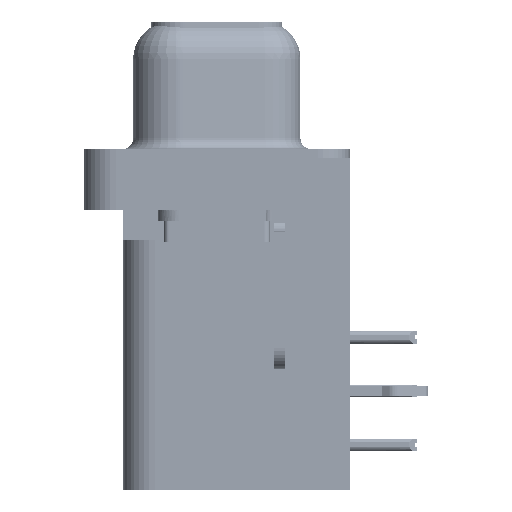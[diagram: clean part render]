
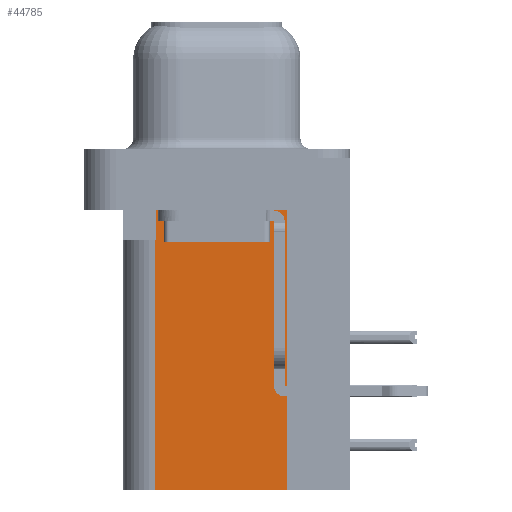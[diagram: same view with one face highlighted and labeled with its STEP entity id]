
A CAD part, left-side view. The second image highlights one B-rep face of the part: STEP entity #44785.
In plain terms, the highlighted planar face has unit normal (-1, 0, 0).
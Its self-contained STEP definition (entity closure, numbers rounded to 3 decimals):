
#141 = AXIS2_PLACEMENT_3D ( 'NONE', #15658, #43529, #22673 ) ;
#3928 = DIRECTION ( 'NONE',  ( 0., 0., -1. ) ) ;
#4712 = DIRECTION ( 'NONE',  ( 0., 1., 0. ) ) ;
#4950 = VERTEX_POINT ( 'NONE', #34825 ) ;
#5890 = VECTOR ( 'NONE', #4712, 1000. ) ;
#6007 = VERTEX_POINT ( 'NONE', #10439 ) ;
#7866 = VERTEX_POINT ( 'NONE', #42041 ) ;
#8659 = LINE ( 'NONE', #20892, #18112 ) ;
#9629 = VERTEX_POINT ( 'NONE', #35778 ) ;
#10373 = ORIENTED_EDGE ( 'NONE', *, *, #26933, .T. ) ;
#10439 = CARTESIAN_POINT ( 'NONE',  ( 3.7, 2.895, -2.5 ) ) ;
#11635 = ORIENTED_EDGE ( 'NONE', *, *, #17318, .F. ) ;
#14782 = DIRECTION ( 'NONE',  ( 0., 1., 0. ) ) ;
#15658 = CARTESIAN_POINT ( 'NONE',  ( 3.7, -3.295, -15.7 ) ) ;
#16443 = LINE ( 'NONE', #43155, #5890 ) ;
#17318 = EDGE_CURVE ( 'NONE', #39804, #7866, #29363, .T. ) ;
#18112 = VECTOR ( 'NONE', #24385, 1000. ) ;
#18471 = ORIENTED_EDGE ( 'NONE', *, *, #22026, .T. ) ;
#19709 = VERTEX_POINT ( 'NONE', #25053 ) ;
#20469 = EDGE_LOOP ( 'NONE', ( #25686, #10373, #35049, #11635, #25827, #18471 ) ) ;
#20892 = CARTESIAN_POINT ( 'NONE',  ( 3.7, -3.295, -2.5 ) ) ;
#21402 = CARTESIAN_POINT ( 'NONE',  ( 3.7, 2.925, -15.7 ) ) ;
#21564 = EDGE_CURVE ( 'NONE', #9629, #39804, #16443, .T. ) ;
#21818 = EDGE_CURVE ( 'NONE', #4950, #6007, #8659, .T. ) ;
#22026 = EDGE_CURVE ( 'NONE', #9629, #4950, #38234, .T. ) ;
#22673 = DIRECTION ( 'NONE',  ( 0., 1., 0. ) ) ;
#22860 = LINE ( 'NONE', #35772, #41390 ) ;
#23137 = FACE_OUTER_BOUND ( 'NONE', #20469, .T. ) ;
#24385 = DIRECTION ( 'NONE',  ( 0., 1., 0. ) ) ;
#25053 = CARTESIAN_POINT ( 'NONE',  ( 3.7, 2.895, -3.9 ) ) ;
#25686 = ORIENTED_EDGE ( 'NONE', *, *, #21818, .T. ) ;
#25827 = ORIENTED_EDGE ( 'NONE', *, *, #21564, .F. ) ;
#26933 = EDGE_CURVE ( 'NONE', #6007, #19709, #31004, .T. ) ;
#28650 = CARTESIAN_POINT ( 'NONE',  ( 3.7, 2.895, -3.9 ) ) ;
#29071 = VECTOR ( 'NONE', #40522, 1000. ) ;
#29363 = LINE ( 'NONE', #21402, #36377 ) ;
#31004 = LINE ( 'NONE', #28650, #40122 ) ;
#32074 = DIRECTION ( 'NONE',  ( 0., 0., 1. ) ) ;
#33429 = EDGE_CURVE ( 'NONE', #19709, #7866, #22860, .T. ) ;
#34825 = CARTESIAN_POINT ( 'NONE',  ( 3.7, -3.295, -2.5 ) ) ;
#35049 = ORIENTED_EDGE ( 'NONE', *, *, #33429, .T. ) ;
#35772 = CARTESIAN_POINT ( 'NONE',  ( 3.7, 0., -3.9 ) ) ;
#35778 = CARTESIAN_POINT ( 'NONE',  ( 3.7, -3.295, -15.7 ) ) ;
#36377 = VECTOR ( 'NONE', #32074, 1000. ) ;
#37075 = CARTESIAN_POINT ( 'NONE',  ( 3.7, -3.295, -15.7 ) ) ;
#38234 = LINE ( 'NONE', #37075, #29071 ) ;
#39804 = VERTEX_POINT ( 'NONE', #40020 ) ;
#40020 = CARTESIAN_POINT ( 'NONE',  ( 3.7, 2.925, -15.7 ) ) ;
#40062 = PLANE ( 'NONE',  #141 ) ;
#40122 = VECTOR ( 'NONE', #3928, 1000. ) ;
#40522 = DIRECTION ( 'NONE',  ( 0., 0., 1. ) ) ;
#41390 = VECTOR ( 'NONE', #14782, 1000. ) ;
#42041 = CARTESIAN_POINT ( 'NONE',  ( 3.7, 2.925, -3.9 ) ) ;
#43155 = CARTESIAN_POINT ( 'NONE',  ( 3.7, -3.295, -15.7 ) ) ;
#43529 = DIRECTION ( 'NONE',  ( 1., 0., 0. ) ) ;
#44785 = ADVANCED_FACE ( 'NONE', ( #23137 ), #40062, .F. ) ;
